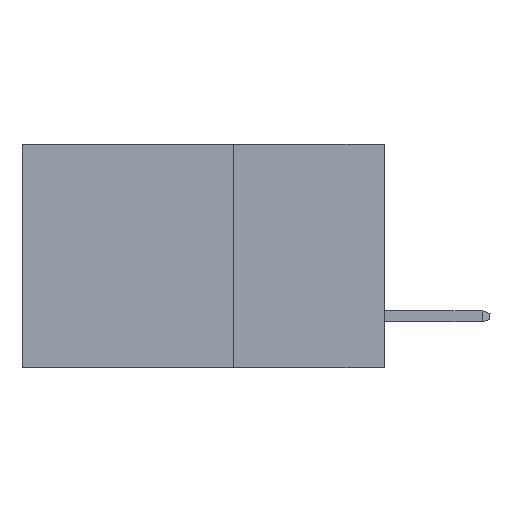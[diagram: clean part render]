
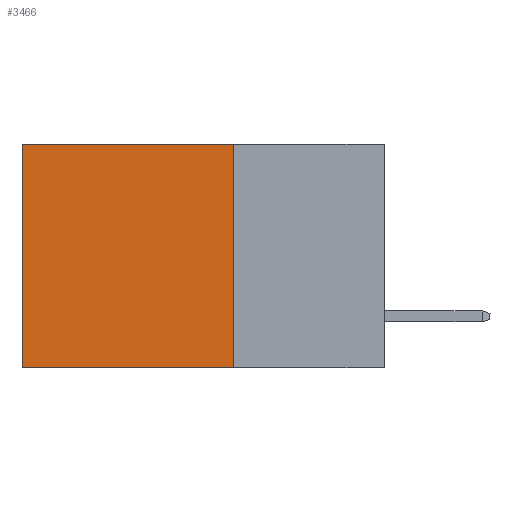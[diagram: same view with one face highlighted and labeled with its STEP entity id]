
A CAD part, left-side view. The second image highlights one B-rep face of the part: STEP entity #3466.
In plain terms, the highlighted planar face has unit normal (-1, 0, 0).
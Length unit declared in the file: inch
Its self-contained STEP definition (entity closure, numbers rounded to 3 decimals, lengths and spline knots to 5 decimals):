
#15 = VERTEX_POINT ( 'NONE', #363 ) ;
#363 = CARTESIAN_POINT ( 'NONE',  ( 0.2615, 0.6, -0.37 ) ) ;
#640 = VECTOR ( 'NONE', #3431, 39.37008 ) ;
#696 = FACE_OUTER_BOUND ( 'NONE', #5544, .T. ) ;
#823 = LINE ( 'NONE', #1543, #640 ) ;
#1543 = CARTESIAN_POINT ( 'NONE',  ( 0.2615, 0.6, -0.37 ) ) ;
#1564 = VECTOR ( 'NONE', #1765, 39.37008 ) ;
#1765 = DIRECTION ( 'NONE',  ( 0., 0., -1. ) ) ;
#1800 = EDGE_CURVE ( 'NONE', #2984, #6042, #4348, .T. ) ;
#2012 = EDGE_CURVE ( 'NONE', #2984, #5123, #2054, .T. ) ;
#2054 = LINE ( 'NONE', #4185, #5121 ) ;
#2324 = CARTESIAN_POINT ( 'NONE',  ( 0.2615, 0.25, 0. ) ) ;
#2442 = CARTESIAN_POINT ( 'NONE',  ( 0.2615, 0.25, -0.37 ) ) ;
#2984 = VERTEX_POINT ( 'NONE', #2324 ) ;
#3431 = DIRECTION ( 'NONE',  ( 0., 0., -1. ) ) ;
#3466 = ADVANCED_FACE ( 'NONE', ( #696 ), #8393, .F. ) ;
#3694 = ORIENTED_EDGE ( 'NONE', *, *, #2012, .T. ) ;
#3724 = EDGE_CURVE ( 'NONE', #5123, #15, #823, .T. ) ;
#3924 = ORIENTED_EDGE ( 'NONE', *, *, #6326, .F. ) ;
#4185 = CARTESIAN_POINT ( 'NONE',  ( 0.2615, 0.25, 0. ) ) ;
#4348 = LINE ( 'NONE', #2442, #1564 ) ;
#4863 = AXIS2_PLACEMENT_3D ( 'NONE', #5132, #7844, #5268 ) ;
#5121 = VECTOR ( 'NONE', #6069, 39.37008 ) ;
#5123 = VERTEX_POINT ( 'NONE', #6197 ) ;
#5132 = CARTESIAN_POINT ( 'NONE',  ( 0.2615, 0.25, -0.37 ) ) ;
#5268 = DIRECTION ( 'NONE',  ( 0., 0., -1. ) ) ;
#5344 = LINE ( 'NONE', #6542, #6922 ) ;
#5544 = EDGE_LOOP ( 'NONE', ( #6652, #3924, #7173, #3694 ) ) ;
#5965 = DIRECTION ( 'NONE',  ( 0., 1., 0. ) ) ;
#6042 = VERTEX_POINT ( 'NONE', #6725 ) ;
#6069 = DIRECTION ( 'NONE',  ( 0., 1., 0. ) ) ;
#6197 = CARTESIAN_POINT ( 'NONE',  ( 0.2615, 0.6, 0. ) ) ;
#6326 = EDGE_CURVE ( 'NONE', #6042, #15, #5344, .T. ) ;
#6542 = CARTESIAN_POINT ( 'NONE',  ( 0.2615, 0.25, -0.37 ) ) ;
#6652 = ORIENTED_EDGE ( 'NONE', *, *, #3724, .T. ) ;
#6725 = CARTESIAN_POINT ( 'NONE',  ( 0.2615, 0.25, -0.37 ) ) ;
#6922 = VECTOR ( 'NONE', #5965, 39.37008 ) ;
#7173 = ORIENTED_EDGE ( 'NONE', *, *, #1800, .F. ) ;
#7844 = DIRECTION ( 'NONE',  ( 1., 0., 0. ) ) ;
#8393 = PLANE ( 'NONE',  #4863 ) ;
